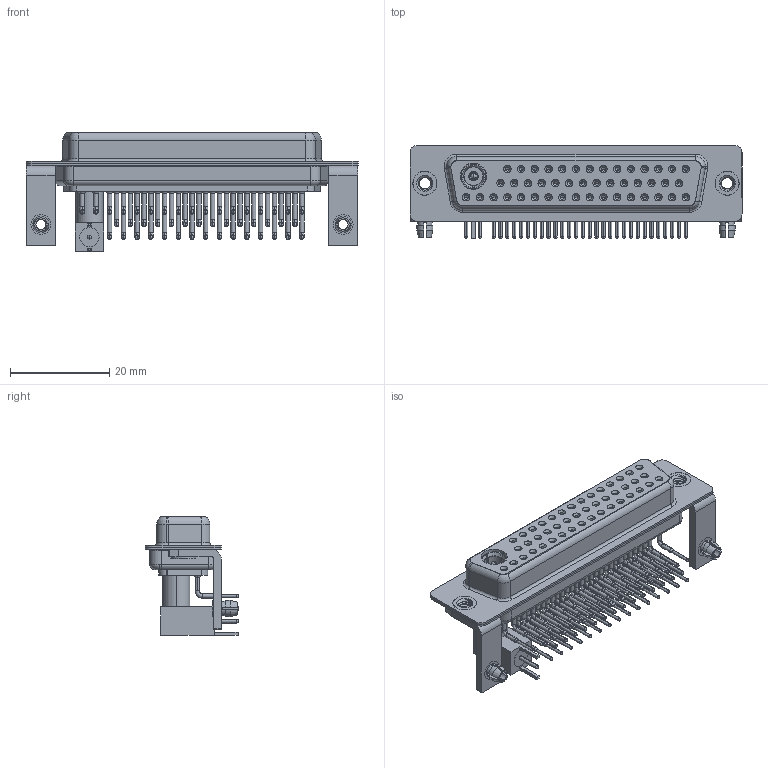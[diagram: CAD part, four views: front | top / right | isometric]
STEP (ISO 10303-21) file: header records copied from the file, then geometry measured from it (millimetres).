
FILE_DESCRIPTION (( 'STEP AP203' ), '1' );
FILE_NAME ('630-47W1240-5T3.STEP', '2022-06-10T08:27:13', ( '' ), ( '' ), 'SwSTEP 2.0', 'SolidWorks 2020', '' );
FILE_SCHEMA (( 'CONFIG_CONTROL_DESIGN' ));
Length unit declared in the file: millimetre
Products named in the file (17): 630Combo Contact Row 1_50 Contacts; Co-Ax Plug_RA 50; 630Combo Contact Row 2_50 Contacts; Insulator RA Pin; Co-Ax Plug Assy_RA 50; 630Combo Stabilizer Bracket_50 Contacts; 630Combo Contact Row 3; 630Combo Threaded Rivet_3; Insulator Pin_Straight PC Tail; 630Combo Board Lock_50 Contacts; Pin_RA 50; Locking Collar; 630Combo Housing_47W1; 630-47W1240-5T3; RA Back Shell_50; 630Combo Shell Rear_50 Contacts; 630Combo Shell Front_50 Contacts
Assembly tree (62 placements, depth 3):
  630-47W1240-5T3
    630Combo Housing_47W1
    630Combo Shell Front_50 Contacts
    630Combo Shell Rear_50 Contacts
    630Combo Threaded Rivet_3  x2
    630Combo Stabilizer Bracket_50 Contacts  x2
    630Combo Board Lock_50 Contacts  x2
    Co-Ax Plug Assy_RA 50
      Co-Ax Plug_RA 50
      Insulator Pin_Straight PC Tail
      Pin_RA 50
      Locking Collar
      RA Back Shell_50
      Insulator RA Pin
    630Combo Contact Row 1_50 Contacts  x15
    630Combo Contact Row 2_50 Contacts  x14
    630Combo Contact Row 3  x17
Bounding box: 67 x 18.8 x 23.95 mm (x, y, z)
Volume: 7896.3 mm3; surface area: 17710.4 mm2
Topology: 61 solids, 61 shells, 3004 faces, 7618 edges, 4800 vertices
Faces by surface type: cylinder 1302, plane 889, cone 555, bspline 191, torus 63, sphere 4
Entity records: 39386 total; most frequent: CARTESIAN_POINT 7873, DIRECTION 6580, ORIENTED_EDGE 5474, AXIS2_PLACEMENT_3D 2737, EDGE_CURVE 2737, VERTEX_POINT 1750, CIRCLE 1502, EDGE_LOOP 1473
